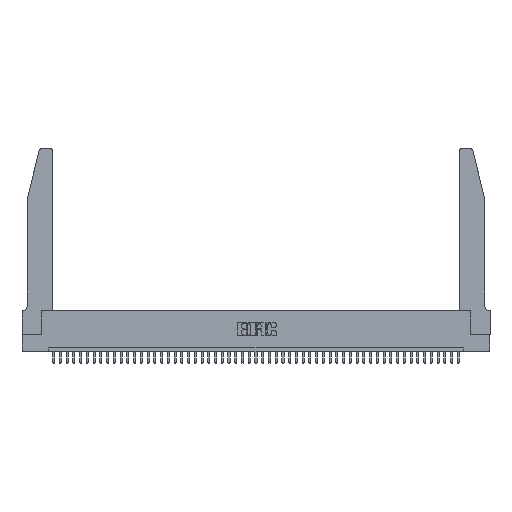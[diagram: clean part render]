
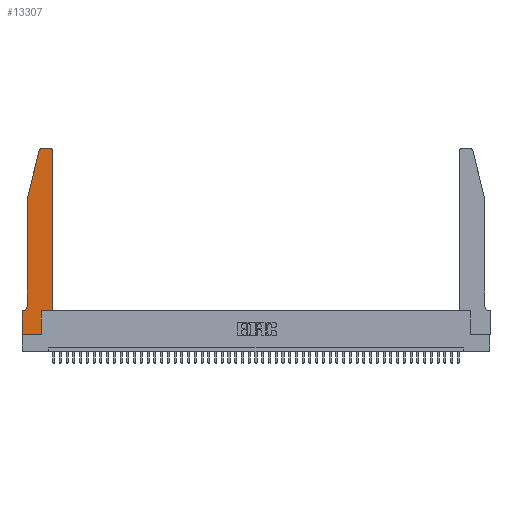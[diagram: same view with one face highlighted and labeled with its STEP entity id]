
A CAD part, top view. The second image highlights one B-rep face of the part: STEP entity #13307.
In plain terms, the highlighted planar face has unit normal (0, 0, 1).
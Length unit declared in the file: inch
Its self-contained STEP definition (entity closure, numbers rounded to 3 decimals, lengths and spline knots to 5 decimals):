
#36 = DIRECTION ( 'NONE',  ( -1., 0., 0. ) ) ;
#329 = EDGE_CURVE ( 'NONE', #42861, #17166, #4313, .T. ) ;
#454 = LINE ( 'NONE', #7279, #18533 ) ;
#498 = CIRCLE ( 'NONE', #18096, 0.07 ) ;
#865 = CARTESIAN_POINT ( 'NONE',  ( 0.0755, 0.42, 0.37 ) ) ;
#1998 = VERTEX_POINT ( 'NONE', #30352 ) ;
#2313 = CARTESIAN_POINT ( 'NONE',  ( 0.4205, 2.72, 0.37 ) ) ;
#2651 = VECTOR ( 'NONE', #36, 39.37008 ) ;
#4019 = LINE ( 'NONE', #13400, #43707 ) ;
#4313 = LINE ( 'NONE', #41055, #2651 ) ;
#4714 = VERTEX_POINT ( 'NONE', #8079 ) ;
#6265 = CARTESIAN_POINT ( 'NONE',  ( 0.0055, 0.42, 0.37 ) ) ;
#6590 = DIRECTION ( 'NONE',  ( 0., 0., -1. ) ) ;
#7279 = CARTESIAN_POINT ( 'NONE',  ( 0.0755, 2., 0.37 ) ) ;
#7441 = DIRECTION ( 'NONE',  ( 1., 0., 0. ) ) ;
#8079 = CARTESIAN_POINT ( 'NONE',  ( 0.4505, 0.35, 0.37 ) ) ;
#8486 = VERTEX_POINT ( 'NONE', #15980 ) ;
#8894 = CARTESIAN_POINT ( 'NONE',  ( 0.4505, 0.35, 0.37 ) ) ;
#9530 = ORIENTED_EDGE ( 'NONE', *, *, #33221, .T. ) ;
#10996 = ORIENTED_EDGE ( 'NONE', *, *, #16047, .T. ) ;
#11254 = VECTOR ( 'NONE', #33805, 39.37008 ) ;
#13307 = ADVANCED_FACE ( 'NONE', ( #16971 ), #25995, .T. ) ;
#13400 = CARTESIAN_POINT ( 'NONE',  ( 0.0755, 2., 0.37 ) ) ;
#13650 = ORIENTED_EDGE ( 'NONE', *, *, #33698, .T. ) ;
#13812 = ORIENTED_EDGE ( 'NONE', *, *, #35422, .T. ) ;
#14196 = LINE ( 'NONE', #34448, #11254 ) ;
#14376 = VERTEX_POINT ( 'NONE', #23658 ) ;
#14466 = VERTEX_POINT ( 'NONE', #20730 ) ;
#14687 = LINE ( 'NONE', #34221, #25202 ) ;
#14885 = CARTESIAN_POINT ( 'NONE',  ( 0., 0.35, 0.37 ) ) ;
#15980 = CARTESIAN_POINT ( 'NONE',  ( 0.2865, 0.35, 0.37 ) ) ;
#16047 = EDGE_CURVE ( 'NONE', #14376, #17827, #37689, .T. ) ;
#16767 = VERTEX_POINT ( 'NONE', #865 ) ;
#16971 = FACE_OUTER_BOUND ( 'NONE', #37987, .T. ) ;
#17166 = VERTEX_POINT ( 'NONE', #27369 ) ;
#17428 = VECTOR ( 'NONE', #43576, 39.37008 ) ;
#17493 = DIRECTION ( 'NONE',  ( -1., 0., 0. ) ) ;
#17827 = VERTEX_POINT ( 'NONE', #42496 ) ;
#17945 = EDGE_CURVE ( 'NONE', #16767, #42861, #498, .T. ) ;
#18096 = AXIS2_PLACEMENT_3D ( 'NONE', #6265, #6590, #17493 ) ;
#18533 = VECTOR ( 'NONE', #33689, 39.37008 ) ;
#19274 = LINE ( 'NONE', #22252, #42032 ) ;
#19853 = CIRCLE ( 'NONE', #21887, 0.03 ) ;
#20730 = CARTESIAN_POINT ( 'NONE',  ( 0.4205, 2.75, 0.37 ) ) ;
#21263 = CARTESIAN_POINT ( 'NONE',  ( 0.2865, 0., 0.37 ) ) ;
#21726 = DIRECTION ( 'NONE',  ( 0., 0., 1. ) ) ;
#21887 = AXIS2_PLACEMENT_3D ( 'NONE', #2313, #32501, #47416 ) ;
#22115 = LINE ( 'NONE', #32226, #17428 ) ;
#22120 = AXIS2_PLACEMENT_3D ( 'NONE', #40818, #21726, #47817 ) ;
#22252 = CARTESIAN_POINT ( 'NONE',  ( 0.4505, 0.35, 0.37 ) ) ;
#23371 = LINE ( 'NONE', #44063, #29880 ) ;
#23658 = CARTESIAN_POINT ( 'NONE',  ( 0.284, 2.75, 0.37 ) ) ;
#25202 = VECTOR ( 'NONE', #30182, 39.37008 ) ;
#25936 = ORIENTED_EDGE ( 'NONE', *, *, #329, .T. ) ;
#25995 = PLANE ( 'NONE',  #45418 ) ;
#27369 = CARTESIAN_POINT ( 'NONE',  ( 0., 0.35, 0.37 ) ) ;
#27549 = DIRECTION ( 'NONE',  ( 0., 1., 0. ) ) ;
#27761 = VECTOR ( 'NONE', #27549, 39.37008 ) ;
#28174 = EDGE_CURVE ( 'NONE', #42282, #8486, #14196, .T. ) ;
#28643 = DIRECTION ( 'NONE',  ( 0., -1., 0. ) ) ;
#28854 = CARTESIAN_POINT ( 'NONE',  ( 0., 0., 0.37 ) ) ;
#28931 = EDGE_CURVE ( 'NONE', #8486, #4714, #19274, .T. ) ;
#29880 = VECTOR ( 'NONE', #30247, 39.37008 ) ;
#30182 = DIRECTION ( 'NONE',  ( 1., 0., 0. ) ) ;
#30225 = ORIENTED_EDGE ( 'NONE', *, *, #28174, .T. ) ;
#30247 = DIRECTION ( 'NONE',  ( 0., -1., 0. ) ) ;
#30352 = CARTESIAN_POINT ( 'NONE',  ( 0.0755, 2., 0.37 ) ) ;
#31056 = ORIENTED_EDGE ( 'NONE', *, *, #41280, .T. ) ;
#31817 = ORIENTED_EDGE ( 'NONE', *, *, #28931, .T. ) ;
#32226 = CARTESIAN_POINT ( 'NONE',  ( 0.2605, 2.75, 0.37 ) ) ;
#32501 = DIRECTION ( 'NONE',  ( 0., 0., 1. ) ) ;
#32989 = VERTEX_POINT ( 'NONE', #28854 ) ;
#33221 = EDGE_CURVE ( 'NONE', #17166, #32989, #23371, .T. ) ;
#33651 = EDGE_CURVE ( 'NONE', #46512, #14466, #19853, .T. ) ;
#33689 = DIRECTION ( 'NONE',  ( -0.239, -0.971, 0. ) ) ;
#33698 = EDGE_CURVE ( 'NONE', #1998, #16767, #4019, .T. ) ;
#33805 = DIRECTION ( 'NONE',  ( 0., 1., 0. ) ) ;
#34221 = CARTESIAN_POINT ( 'NONE',  ( 0., 0., 0.37 ) ) ;
#34448 = CARTESIAN_POINT ( 'NONE',  ( 0.2865, 0.35, 0.37 ) ) ;
#35422 = EDGE_CURVE ( 'NONE', #17827, #1998, #454, .T. ) ;
#36297 = ORIENTED_EDGE ( 'NONE', *, *, #33651, .T. ) ;
#36776 = EDGE_CURVE ( 'NONE', #32989, #42282, #14687, .T. ) ;
#37621 = LINE ( 'NONE', #8894, #27761 ) ;
#37689 = CIRCLE ( 'NONE', #22120, 0.03 ) ;
#37987 = EDGE_LOOP ( 'NONE', ( #47563, #10996, #13812, #13650, #43639, #25936, #9530, #46397, #30225, #31817, #31056, #36297 ) ) ;
#38341 = DIRECTION ( 'NONE',  ( 1., 0., 0. ) ) ;
#39863 = CARTESIAN_POINT ( 'NONE',  ( 0.4505, 2.72, 0.37 ) ) ;
#40818 = CARTESIAN_POINT ( 'NONE',  ( 0.284, 2.72, 0.37 ) ) ;
#40940 = DIRECTION ( 'NONE',  ( 0., 0., 1. ) ) ;
#41055 = CARTESIAN_POINT ( 'NONE',  ( 0.0755, 0.35, 0.37 ) ) ;
#41280 = EDGE_CURVE ( 'NONE', #4714, #46512, #37621, .T. ) ;
#42020 = CARTESIAN_POINT ( 'NONE',  ( 0.0055, 0.35, 0.37 ) ) ;
#42032 = VECTOR ( 'NONE', #7441, 39.37008 ) ;
#42282 = VERTEX_POINT ( 'NONE', #21263 ) ;
#42496 = CARTESIAN_POINT ( 'NONE',  ( 0.25487, 2.72718, 0.37 ) ) ;
#42861 = VERTEX_POINT ( 'NONE', #42020 ) ;
#43576 = DIRECTION ( 'NONE',  ( -1., 0., 0. ) ) ;
#43639 = ORIENTED_EDGE ( 'NONE', *, *, #17945, .T. ) ;
#43707 = VECTOR ( 'NONE', #28643, 39.37008 ) ;
#44063 = CARTESIAN_POINT ( 'NONE',  ( 0., 0., 0.37 ) ) ;
#45418 = AXIS2_PLACEMENT_3D ( 'NONE', #14885, #40940, #38341 ) ;
#45540 = EDGE_CURVE ( 'NONE', #14466, #14376, #22115, .T. ) ;
#46397 = ORIENTED_EDGE ( 'NONE', *, *, #36776, .T. ) ;
#46512 = VERTEX_POINT ( 'NONE', #39863 ) ;
#47416 = DIRECTION ( 'NONE',  ( 1., 0., 0. ) ) ;
#47563 = ORIENTED_EDGE ( 'NONE', *, *, #45540, .T. ) ;
#47817 = DIRECTION ( 'NONE',  ( 1., 0., 0. ) ) ;
